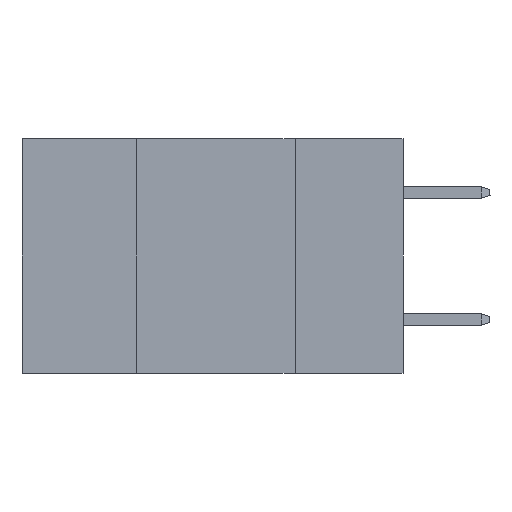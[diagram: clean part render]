
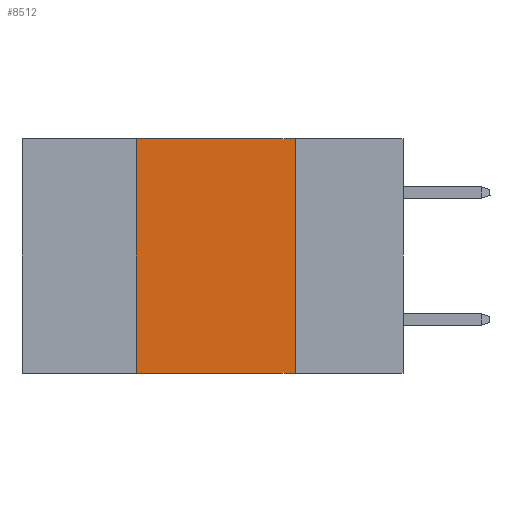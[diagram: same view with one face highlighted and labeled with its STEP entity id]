
A CAD part, left-side view. The second image highlights one B-rep face of the part: STEP entity #8512.
In plain terms, the highlighted planar face has unit normal (-1, 0, 0).
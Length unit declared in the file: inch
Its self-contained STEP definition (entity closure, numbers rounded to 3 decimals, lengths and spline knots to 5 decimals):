
#393 = AXIS2_PLACEMENT_3D ( 'NONE', #5480, #2983, #564 ) ;
#564 = DIRECTION ( 'NONE',  ( 0., 0., -1. ) ) ;
#1003 = CARTESIAN_POINT ( 'NONE',  ( 0., 0.17, -0.37 ) ) ;
#1005 = VECTOR ( 'NONE', #13259, 39.37008 ) ;
#1374 = EDGE_CURVE ( 'NONE', #11500, #3595, #8629, .T. ) ;
#2159 = EDGE_CURVE ( 'NONE', #12364, #4812, #4665, .T. ) ;
#2326 = CARTESIAN_POINT ( 'NONE',  ( 0., 0.42, 0. ) ) ;
#2983 = DIRECTION ( 'NONE',  ( 1., 0., 0. ) ) ;
#3340 = CARTESIAN_POINT ( 'NONE',  ( 0., 0.42, 0. ) ) ;
#3595 = VERTEX_POINT ( 'NONE', #6219 ) ;
#4502 = ORIENTED_EDGE ( 'NONE', *, *, #2159, .T. ) ;
#4665 = LINE ( 'NONE', #14737, #1005 ) ;
#4812 = VERTEX_POINT ( 'NONE', #1003 ) ;
#5480 = CARTESIAN_POINT ( 'NONE',  ( 0., 0.6, 0. ) ) ;
#5589 = EDGE_LOOP ( 'NONE', ( #12998, #8413, #6802, #4502 ) ) ;
#6023 = VECTOR ( 'NONE', #9732, 39.37008 ) ;
#6219 = CARTESIAN_POINT ( 'NONE',  ( 0., 0.17, 0. ) ) ;
#6605 = CARTESIAN_POINT ( 'NONE',  ( 0., 0.6, 0. ) ) ;
#6802 = ORIENTED_EDGE ( 'NONE', *, *, #15445, .F. ) ;
#7338 = DIRECTION ( 'NONE',  ( 0., 0., 1. ) ) ;
#8063 = FACE_OUTER_BOUND ( 'NONE', #5589, .T. ) ;
#8413 = ORIENTED_EDGE ( 'NONE', *, *, #1374, .F. ) ;
#8512 = ADVANCED_FACE ( 'NONE', ( #8063 ), #11822, .F. ) ;
#8629 = LINE ( 'NONE', #6605, #11480 ) ;
#9208 = CARTESIAN_POINT ( 'NONE',  ( 0., 0.42, -0.37 ) ) ;
#9732 = DIRECTION ( 'NONE',  ( 0., 0., -1. ) ) ;
#10877 = LINE ( 'NONE', #14576, #6023 ) ;
#11480 = VECTOR ( 'NONE', #11486, 39.37008 ) ;
#11486 = DIRECTION ( 'NONE',  ( 0., -1., 0. ) ) ;
#11500 = VERTEX_POINT ( 'NONE', #3340 ) ;
#11822 = PLANE ( 'NONE',  #393 ) ;
#12364 = VERTEX_POINT ( 'NONE', #9208 ) ;
#12885 = EDGE_CURVE ( 'NONE', #3595, #4812, #10877, .T. ) ;
#12998 = ORIENTED_EDGE ( 'NONE', *, *, #12885, .F. ) ;
#13142 = VECTOR ( 'NONE', #7338, 39.37008 ) ;
#13259 = DIRECTION ( 'NONE',  ( 0., -1., 0. ) ) ;
#13566 = LINE ( 'NONE', #2326, #13142 ) ;
#14576 = CARTESIAN_POINT ( 'NONE',  ( 0., 0.17, 0. ) ) ;
#14737 = CARTESIAN_POINT ( 'NONE',  ( 0., 0.6, -0.37 ) ) ;
#15445 = EDGE_CURVE ( 'NONE', #12364, #11500, #13566, .T. ) ;
